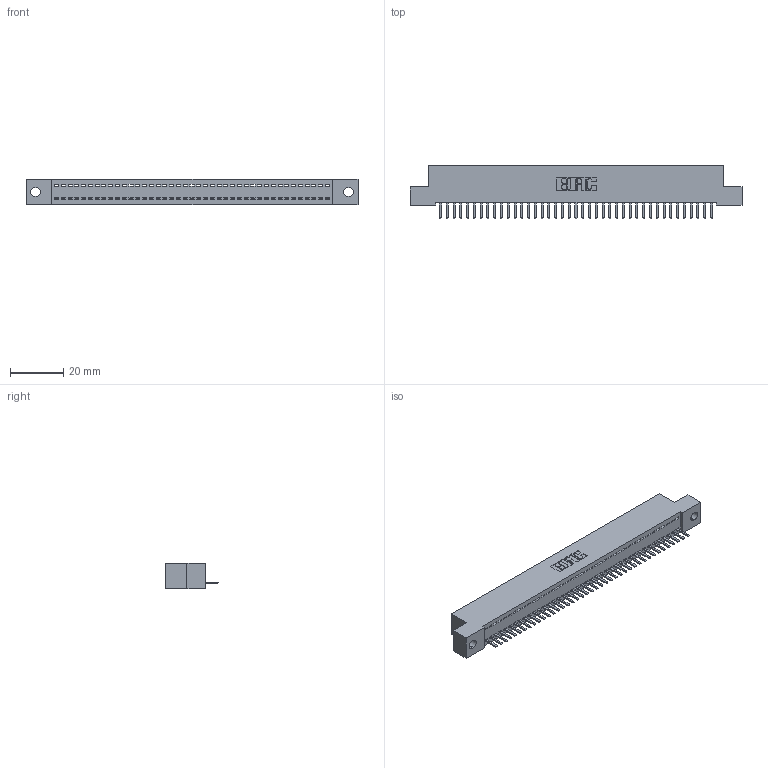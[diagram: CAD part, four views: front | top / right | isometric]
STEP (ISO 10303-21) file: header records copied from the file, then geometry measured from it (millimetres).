
FILE_DESCRIPTION (( 'STEP AP203' ), '1' );
FILE_NAME ('392-041-520-102.STEP', '2019-10-07T20:24:27', ( '' ), ( '' ), 'SwSTEP 2.0', 'SolidWorks 2016', '' );
FILE_SCHEMA (( 'CONFIG_CONTROL_DESIGN' ));
Length unit declared in the file: inch
Products named in the file (3): 342 Part_.128 Slot; 345-292-001_345-293-120; 392-041-520-102
Assembly tree (42 placements, depth 2):
  392-041-520-102
    342 Part_.128 Slot
    345-292-001_345-293-120  x41
Bounding box: 124.46 x 20.02 x 9.4 mm (x, y, z)
Volume: 10738.9 mm3; surface area: 15133.3 mm2
Topology: 42 solids, 42 shells, 2656 faces, 7855 edges, 5126 vertices
Faces by surface type: plane 1874, cylinder 782
Entity records: 25311 total; most frequent: CARTESIAN_POINT 4385, ORIENTED_EDGE 4350, DIRECTION 3689, EDGE_CURVE 2175, LINE 2043, VECTOR 2043, VERTEX_POINT 1446, AXIS2_PLACEMENT_3D 823
